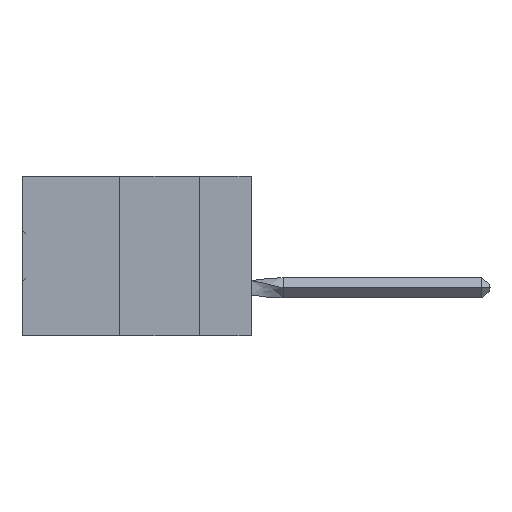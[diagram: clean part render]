
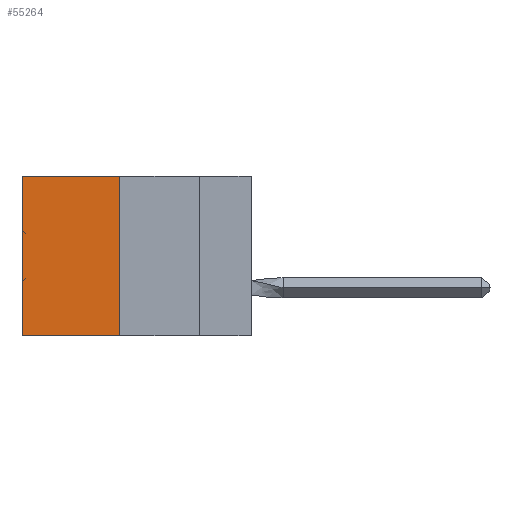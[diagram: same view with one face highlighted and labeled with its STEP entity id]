
A CAD part, left-side view. The second image highlights one B-rep face of the part: STEP entity #55264.
In plain terms, the highlighted planar face has unit normal (-1, 0, 0).
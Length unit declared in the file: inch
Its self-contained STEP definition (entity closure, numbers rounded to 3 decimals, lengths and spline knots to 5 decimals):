
#2106 = CARTESIAN_POINT ( 'NONE',  ( 0.305, 0.413, -0.5 ) ) ;
#2150 = VERTEX_POINT ( 'NONE', #39894 ) ;
#4097 = EDGE_CURVE ( 'NONE', #8435, #27664, #18181, .T. ) ;
#7452 = CARTESIAN_POINT ( 'NONE',  ( 0.305, 0.413, -0.5 ) ) ;
#7870 = VECTOR ( 'NONE', #26316, 39.37008 ) ;
#8435 = VERTEX_POINT ( 'NONE', #2106 ) ;
#11863 = ORIENTED_EDGE ( 'NONE', *, *, #46194, .T. ) ;
#14438 = ORIENTED_EDGE ( 'NONE', *, *, #4097, .F. ) ;
#18181 = LINE ( 'NONE', #58089, #57047 ) ;
#21582 = DIRECTION ( 'NONE',  ( 0., 0., -1. ) ) ;
#23925 = LINE ( 'NONE', #57273, #60497 ) ;
#26316 = DIRECTION ( 'NONE',  ( 0., 0., -1. ) ) ;
#26735 = DIRECTION ( 'NONE',  ( 1., 0., 0. ) ) ;
#27664 = VERTEX_POINT ( 'NONE', #35519 ) ;
#29645 = CARTESIAN_POINT ( 'NONE',  ( 0.305, 0.72, -0.5 ) ) ;
#32211 = VERTEX_POINT ( 'NONE', #58972 ) ;
#34293 = EDGE_LOOP ( 'NONE', ( #11863, #14438, #46708, #38755 ) ) ;
#34349 = DIRECTION ( 'NONE',  ( 0., 0., -1. ) ) ;
#35519 = CARTESIAN_POINT ( 'NONE',  ( 0.305, 0.72, -0.5 ) ) ;
#35651 = VECTOR ( 'NONE', #34349, 39.37008 ) ;
#36942 = FACE_OUTER_BOUND ( 'NONE', #34293, .T. ) ;
#37846 = DIRECTION ( 'NONE',  ( 0., 1., 0. ) ) ;
#38392 = AXIS2_PLACEMENT_3D ( 'NONE', #7452, #26735, #21582 ) ;
#38590 = LINE ( 'NONE', #29645, #35651 ) ;
#38755 = ORIENTED_EDGE ( 'NONE', *, *, #59425, .T. ) ;
#38869 = DIRECTION ( 'NONE',  ( 0., 1., 0. ) ) ;
#39894 = CARTESIAN_POINT ( 'NONE',  ( 0.305, 0.72, 0. ) ) ;
#40778 = CARTESIAN_POINT ( 'NONE',  ( 0.305, 0.413, -0.5 ) ) ;
#46194 = EDGE_CURVE ( 'NONE', #2150, #27664, #38590, .T. ) ;
#46708 = ORIENTED_EDGE ( 'NONE', *, *, #58475, .F. ) ;
#49628 = PLANE ( 'NONE',  #38392 ) ;
#55264 = ADVANCED_FACE ( 'NONE', ( #36942 ), #49628, .F. ) ;
#56973 = LINE ( 'NONE', #40778, #7870 ) ;
#57047 = VECTOR ( 'NONE', #38869, 39.37008 ) ;
#57273 = CARTESIAN_POINT ( 'NONE',  ( 0.305, 0.413, 0. ) ) ;
#58089 = CARTESIAN_POINT ( 'NONE',  ( 0.305, 0.413, -0.5 ) ) ;
#58475 = EDGE_CURVE ( 'NONE', #32211, #8435, #56973, .T. ) ;
#58972 = CARTESIAN_POINT ( 'NONE',  ( 0.305, 0.413, 0. ) ) ;
#59425 = EDGE_CURVE ( 'NONE', #32211, #2150, #23925, .T. ) ;
#60497 = VECTOR ( 'NONE', #37846, 39.37008 ) ;
